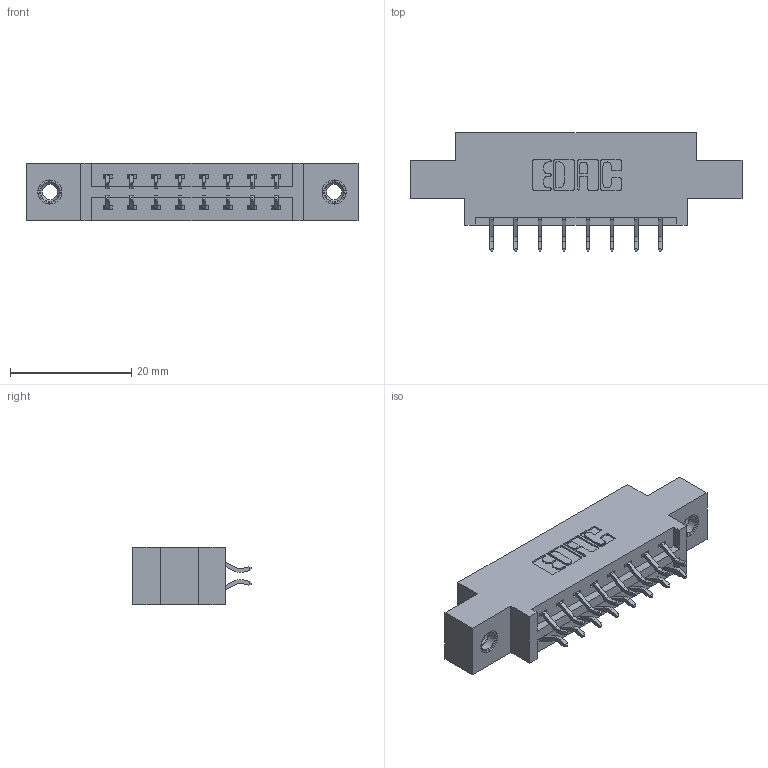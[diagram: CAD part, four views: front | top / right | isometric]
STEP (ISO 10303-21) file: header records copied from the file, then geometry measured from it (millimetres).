
FILE_DESCRIPTION (( 'STEP AP203' ), '1' );
FILE_NAME ('387-016-556-807.STEP', '2018-09-11T12:12:10', ( '' ), ( '' ), 'SwSTEP 2.0', 'SolidWorks 2016', '' );
FILE_SCHEMA (( 'CONFIG_CONTROL_DESIGN' ));
Length unit declared in the file: inch
Products named in the file (4): 345-250-001_345-250-005-103; 387-016-556-807; 337 Part_0.170 Offset - 0.156 Dia-TI; 345-292-001_556 Tail
Assembly tree (19 placements, depth 2):
  387-016-556-807
    337 Part_0.170 Offset - 0.156 Dia-TI
    345-292-001_556 Tail  x16
    345-250-001_345-250-005-103  x2
Bounding box: 54.71 x 19.57 x 9.4 mm (x, y, z)
Volume: 5181.7 mm3; surface area: 5654.6 mm2
Topology: 19 solids, 19 shells, 1138 faces, 3323 edges, 2186 vertices
Faces by surface type: plane 778, cylinder 344, cone 12, torus 4
Entity records: 12138 total; most frequent: CARTESIAN_POINT 2069, ORIENTED_EDGE 1986, DIRECTION 1843, EDGE_CURVE 993, VECTOR 837, LINE 837, VERTEX_POINT 656, AXIS2_PLACEMENT_3D 503
